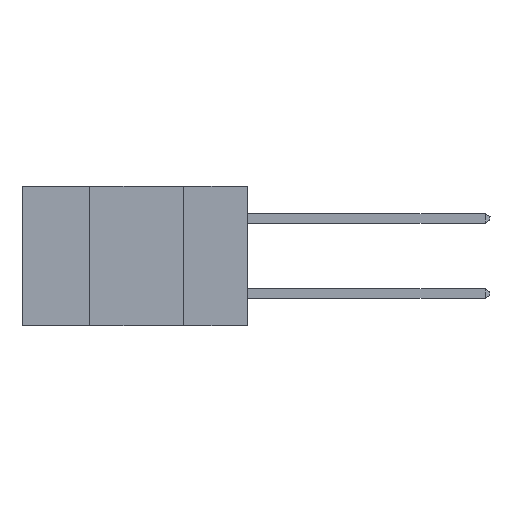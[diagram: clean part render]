
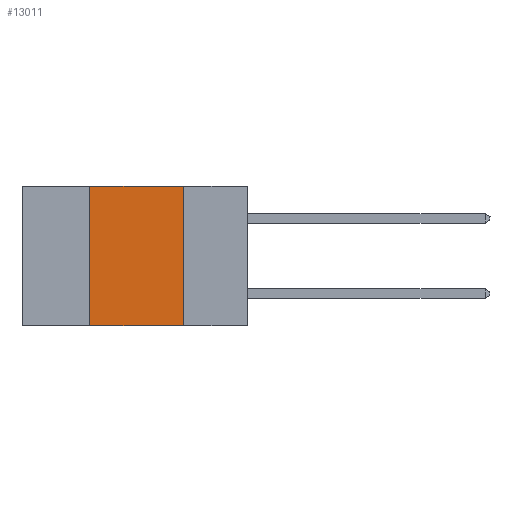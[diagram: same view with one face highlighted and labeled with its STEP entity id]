
A CAD part, left-side view. The second image highlights one B-rep face of the part: STEP entity #13011.
In plain terms, the highlighted planar face has unit normal (-1, 0, 0).
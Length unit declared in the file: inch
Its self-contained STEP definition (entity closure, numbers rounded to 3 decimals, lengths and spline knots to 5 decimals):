
#781 = LINE ( 'NONE', #8524, #17004 ) ;
#1028 = DIRECTION ( 'NONE',  ( 0., -1., 0. ) ) ;
#1576 = PLANE ( 'NONE',  #9363 ) ;
#1653 = CARTESIAN_POINT ( 'NONE',  ( 0., 0.42, -0.37 ) ) ;
#1818 = VERTEX_POINT ( 'NONE', #17570 ) ;
#2214 = CARTESIAN_POINT ( 'NONE',  ( 0., 0.6, 0. ) ) ;
#2385 = LINE ( 'NONE', #13919, #12566 ) ;
#2463 = VERTEX_POINT ( 'NONE', #16279 ) ;
#2852 = DIRECTION ( 'NONE',  ( 1., 0., 0. ) ) ;
#3256 = EDGE_CURVE ( 'NONE', #1818, #4370, #15486, .T. ) ;
#3400 = VECTOR ( 'NONE', #1028, 39.37008 ) ;
#4342 = EDGE_LOOP ( 'NONE', ( #8116, #15231, #11244, #15157 ) ) ;
#4370 = VERTEX_POINT ( 'NONE', #16691 ) ;
#5545 = DIRECTION ( 'NONE',  ( 0., 0., -1. ) ) ;
#5708 = VECTOR ( 'NONE', #16182, 39.37008 ) ;
#5951 = CARTESIAN_POINT ( 'NONE',  ( 0., 0.17, -0.37 ) ) ;
#7621 = VERTEX_POINT ( 'NONE', #5951 ) ;
#8116 = ORIENTED_EDGE ( 'NONE', *, *, #9090, .F. ) ;
#8524 = CARTESIAN_POINT ( 'NONE',  ( 0., 0.17, -0.37 ) ) ;
#9090 = EDGE_CURVE ( 'NONE', #4370, #7621, #781, .T. ) ;
#9363 = AXIS2_PLACEMENT_3D ( 'NONE', #17847, #2852, #16015 ) ;
#11244 = ORIENTED_EDGE ( 'NONE', *, *, #14767, .F. ) ;
#12566 = VECTOR ( 'NONE', #15274, 39.37008 ) ;
#13011 = ADVANCED_FACE ( 'NONE', ( #17566 ), #1576, .F. ) ;
#13919 = CARTESIAN_POINT ( 'NONE',  ( 0., 0.6, -0.37 ) ) ;
#14767 = EDGE_CURVE ( 'NONE', #2463, #1818, #17454, .T. ) ;
#15157 = ORIENTED_EDGE ( 'NONE', *, *, #17241, .T. ) ;
#15231 = ORIENTED_EDGE ( 'NONE', *, *, #3256, .F. ) ;
#15274 = DIRECTION ( 'NONE',  ( 0., -1., 0. ) ) ;
#15486 = LINE ( 'NONE', #2214, #3400 ) ;
#16015 = DIRECTION ( 'NONE',  ( 0., 0., -1. ) ) ;
#16182 = DIRECTION ( 'NONE',  ( 0., 0., 1. ) ) ;
#16279 = CARTESIAN_POINT ( 'NONE',  ( 0., 0.42, -0.37 ) ) ;
#16691 = CARTESIAN_POINT ( 'NONE',  ( 0., 0.17, 0. ) ) ;
#17004 = VECTOR ( 'NONE', #5545, 39.37008 ) ;
#17241 = EDGE_CURVE ( 'NONE', #2463, #7621, #2385, .T. ) ;
#17454 = LINE ( 'NONE', #1653, #5708 ) ;
#17566 = FACE_OUTER_BOUND ( 'NONE', #4342, .T. ) ;
#17570 = CARTESIAN_POINT ( 'NONE',  ( 0., 0.42, 0. ) ) ;
#17847 = CARTESIAN_POINT ( 'NONE',  ( 0., 0.6, 0. ) ) ;
